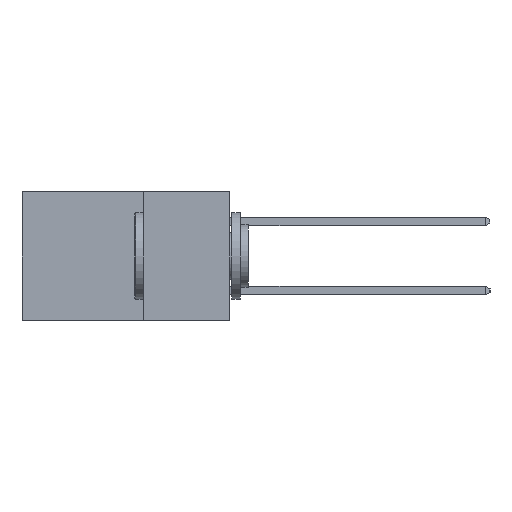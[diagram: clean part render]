
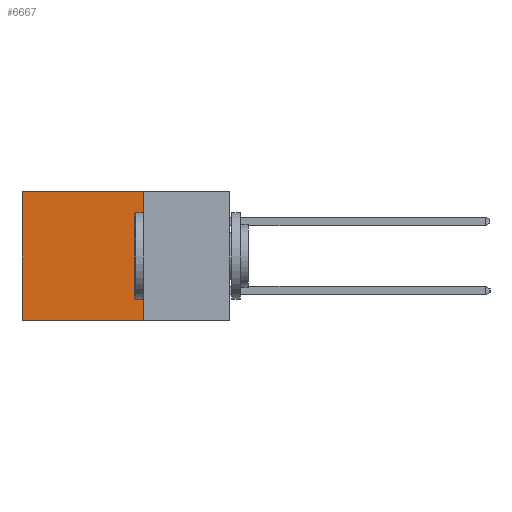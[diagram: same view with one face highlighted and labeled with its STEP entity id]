
A CAD part, left-side view. The second image highlights one B-rep face of the part: STEP entity #6667.
In plain terms, the highlighted planar face has unit normal (-1, 0, 0).
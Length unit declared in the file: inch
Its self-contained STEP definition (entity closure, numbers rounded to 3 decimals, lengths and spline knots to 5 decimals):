
#288 = VECTOR ( 'NONE', #3578, 39.37008 ) ;
#569 = CARTESIAN_POINT ( 'NONE',  ( 0.2615, 0.25, -0.37 ) ) ;
#1128 = CARTESIAN_POINT ( 'NONE',  ( 0.2615, 0.25, -0.37 ) ) ;
#1395 = ORIENTED_EDGE ( 'NONE', *, *, #10095, .T. ) ;
#1837 = VECTOR ( 'NONE', #15597, 39.37008 ) ;
#2898 = EDGE_CURVE ( 'NONE', #11716, #11560, #6839, .T. ) ;
#3578 = DIRECTION ( 'NONE',  ( 0., 1., 0. ) ) ;
#3707 = CARTESIAN_POINT ( 'NONE',  ( 0.2615, 0.25, 0. ) ) ;
#4064 = LINE ( 'NONE', #3707, #288 ) ;
#4214 = CARTESIAN_POINT ( 'NONE',  ( 0.2615, 0.6, -0.37 ) ) ;
#4942 = ORIENTED_EDGE ( 'NONE', *, *, #11844, .T. ) ;
#5042 = EDGE_CURVE ( 'NONE', #7535, #11716, #6515, .T. ) ;
#5192 = LINE ( 'NONE', #4214, #1837 ) ;
#5386 = PLANE ( 'NONE',  #7467 ) ;
#5515 = DIRECTION ( 'NONE',  ( 0., 0., -1. ) ) ;
#5668 = CARTESIAN_POINT ( 'NONE',  ( 0.2615, 0.25, -0.37 ) ) ;
#5937 = ORIENTED_EDGE ( 'NONE', *, *, #5042, .F. ) ;
#6366 = VECTOR ( 'NONE', #9684, 39.37008 ) ;
#6515 = LINE ( 'NONE', #5668, #17221 ) ;
#6667 = ADVANCED_FACE ( 'NONE', ( #7424 ), #5386, .F. ) ;
#6839 = LINE ( 'NONE', #6898, #6366 ) ;
#6898 = CARTESIAN_POINT ( 'NONE',  ( 0.2615, 0.25, -0.37 ) ) ;
#7424 = FACE_OUTER_BOUND ( 'NONE', #16243, .T. ) ;
#7467 = AXIS2_PLACEMENT_3D ( 'NONE', #569, #9426, #12962 ) ;
#7535 = VERTEX_POINT ( 'NONE', #14185 ) ;
#8350 = ORIENTED_EDGE ( 'NONE', *, *, #2898, .F. ) ;
#9426 = DIRECTION ( 'NONE',  ( 1., 0., 0. ) ) ;
#9484 = CARTESIAN_POINT ( 'NONE',  ( 0.2615, 0.6, -0.37 ) ) ;
#9684 = DIRECTION ( 'NONE',  ( 0., 1., 0. ) ) ;
#10095 = EDGE_CURVE ( 'NONE', #7535, #15942, #4064, .T. ) ;
#11560 = VERTEX_POINT ( 'NONE', #9484 ) ;
#11716 = VERTEX_POINT ( 'NONE', #1128 ) ;
#11844 = EDGE_CURVE ( 'NONE', #15942, #11560, #5192, .T. ) ;
#12962 = DIRECTION ( 'NONE',  ( 0., 0., -1. ) ) ;
#14185 = CARTESIAN_POINT ( 'NONE',  ( 0.2615, 0.25, 0. ) ) ;
#14278 = CARTESIAN_POINT ( 'NONE',  ( 0.2615, 0.6, 0. ) ) ;
#15597 = DIRECTION ( 'NONE',  ( 0., 0., -1. ) ) ;
#15942 = VERTEX_POINT ( 'NONE', #14278 ) ;
#16243 = EDGE_LOOP ( 'NONE', ( #4942, #8350, #5937, #1395 ) ) ;
#17221 = VECTOR ( 'NONE', #5515, 39.37008 ) ;
